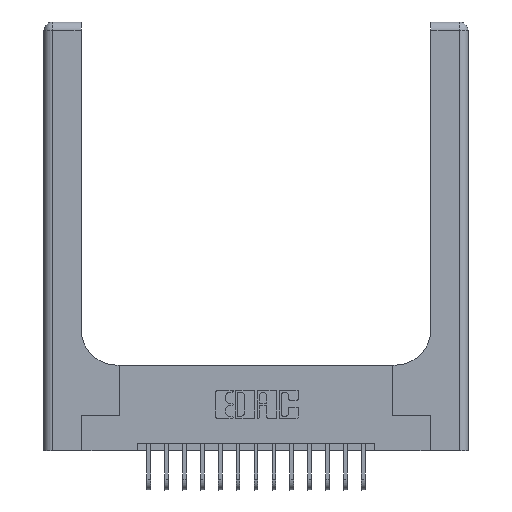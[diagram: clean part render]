
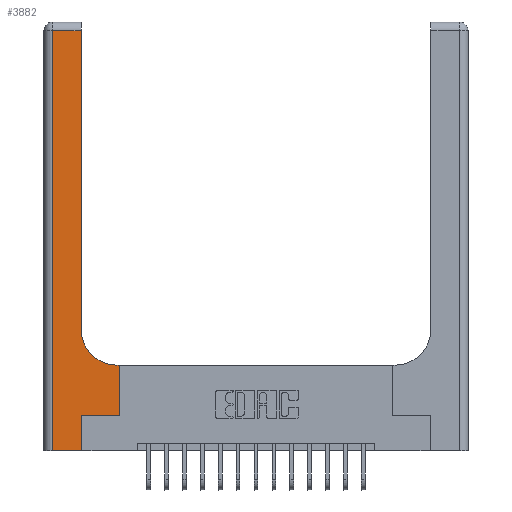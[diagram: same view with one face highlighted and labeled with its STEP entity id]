
A CAD part, top view. The second image highlights one B-rep face of the part: STEP entity #3882.
In plain terms, the highlighted planar face has unit normal (0, 0, 1).
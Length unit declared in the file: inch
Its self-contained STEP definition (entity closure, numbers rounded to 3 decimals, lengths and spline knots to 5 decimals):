
#347 = LINE ( 'NONE', #11048, #7003 ) ;
#745 = DIRECTION ( 'NONE',  ( 0., 0., -1. ) ) ;
#1070 = VERTEX_POINT ( 'NONE', #12619 ) ;
#1079 = VERTEX_POINT ( 'NONE', #16019 ) ;
#1255 = DIRECTION ( 'NONE',  ( 0., 1., 0. ) ) ;
#1820 = DIRECTION ( 'NONE',  ( 0., 0., -1. ) ) ;
#1949 = VECTOR ( 'NONE', #17035, 39.37008 ) ;
#2399 = CARTESIAN_POINT ( 'NONE',  ( 0.265, 0., 0.37 ) ) ;
#2413 = CARTESIAN_POINT ( 'NONE',  ( 0.06, 0., 0.37 ) ) ;
#2443 = EDGE_CURVE ( 'NONE', #8974, #7378, #15107, .T. ) ;
#2961 = DIRECTION ( 'NONE',  ( 0., 1., 0. ) ) ;
#3458 = DIRECTION ( 'NONE',  ( 0., -1., 0. ) ) ;
#3665 = EDGE_CURVE ( 'NONE', #13594, #1070, #16737, .T. ) ;
#3882 = ADVANCED_FACE ( 'NONE', ( #6750 ), #15320, .F. ) ;
#3956 = VECTOR ( 'NONE', #4130, 39.37008 ) ;
#4108 = ORIENTED_EDGE ( 'NONE', *, *, #6225, .T. ) ;
#4130 = DIRECTION ( 'NONE',  ( 1., 0., 0. ) ) ;
#4310 = EDGE_CURVE ( 'NONE', #1079, #11461, #16512, .T. ) ;
#4519 = ORIENTED_EDGE ( 'NONE', *, *, #4310, .T. ) ;
#4709 = ORIENTED_EDGE ( 'NONE', *, *, #11155, .T. ) ;
#5202 = EDGE_CURVE ( 'NONE', #15884, #7042, #11118, .T. ) ;
#5296 = AXIS2_PLACEMENT_3D ( 'NONE', #7367, #745, #10072 ) ;
#5558 = ORIENTED_EDGE ( 'NONE', *, *, #5202, .T. ) ;
#6225 = EDGE_CURVE ( 'NONE', #1070, #1079, #11086, .T. ) ;
#6324 = CARTESIAN_POINT ( 'NONE',  ( 0.26, 0.85, 0.37 ) ) ;
#6667 = VECTOR ( 'NONE', #8666, 39.37008 ) ;
#6750 = FACE_OUTER_BOUND ( 'NONE', #10823, .T. ) ;
#6798 = ORIENTED_EDGE ( 'NONE', *, *, #9149, .T. ) ;
#7003 = VECTOR ( 'NONE', #12362, 39.37008 ) ;
#7042 = VERTEX_POINT ( 'NONE', #2413 ) ;
#7367 = CARTESIAN_POINT ( 'NONE',  ( 0., 3., 0.37 ) ) ;
#7378 = VERTEX_POINT ( 'NONE', #12519 ) ;
#7526 = VECTOR ( 'NONE', #3458, 39.37008 ) ;
#8053 = VECTOR ( 'NONE', #1255, 39.37008 ) ;
#8268 = CARTESIAN_POINT ( 'NONE',  ( 0.528, 0.25, 0.37 ) ) ;
#8422 = CARTESIAN_POINT ( 'NONE',  ( 0.06, 2.94, 0.37 ) ) ;
#8666 = DIRECTION ( 'NONE',  ( -1., 0., 0. ) ) ;
#8974 = VERTEX_POINT ( 'NONE', #2399 ) ;
#9086 = CARTESIAN_POINT ( 'NONE',  ( 0., 0., 0.37 ) ) ;
#9149 = EDGE_CURVE ( 'NONE', #7378, #13594, #14131, .T. ) ;
#9816 = CARTESIAN_POINT ( 'NONE',  ( 0.51, 0.85, 0.37 ) ) ;
#10072 = DIRECTION ( 'NONE',  ( -1., 0., 0. ) ) ;
#10255 = VERTEX_POINT ( 'NONE', #16000 ) ;
#10607 = EDGE_CURVE ( 'NONE', #10255, #15884, #347, .T. ) ;
#10615 = CARTESIAN_POINT ( 'NONE',  ( 0.265, 0., 0.37 ) ) ;
#10823 = EDGE_LOOP ( 'NONE', ( #4709, #15743, #5558, #13059, #16574, #6798, #14280, #4108, #4519 ) ) ;
#11048 = CARTESIAN_POINT ( 'NONE',  ( 0., 2.94, 0.37 ) ) ;
#11086 = LINE ( 'NONE', #13944, #6667 ) ;
#11118 = LINE ( 'NONE', #16694, #7526 ) ;
#11155 = EDGE_CURVE ( 'NONE', #11461, #10255, #12835, .T. ) ;
#11175 = DIRECTION ( 'NONE',  ( 1., 0., 0. ) ) ;
#11461 = VERTEX_POINT ( 'NONE', #6324 ) ;
#12117 = CARTESIAN_POINT ( 'NONE',  ( 0.265, 0.25, 0.37 ) ) ;
#12124 = AXIS2_PLACEMENT_3D ( 'NONE', #9816, #1820, #11175 ) ;
#12362 = DIRECTION ( 'NONE',  ( -1., 0., 0. ) ) ;
#12519 = CARTESIAN_POINT ( 'NONE',  ( 0.265, 0.25, 0.37 ) ) ;
#12619 = CARTESIAN_POINT ( 'NONE',  ( 0.528, 0.6, 0.37 ) ) ;
#12835 = LINE ( 'NONE', #13605, #15508 ) ;
#13059 = ORIENTED_EDGE ( 'NONE', *, *, #13138, .T. ) ;
#13138 = EDGE_CURVE ( 'NONE', #7042, #8974, #16109, .T. ) ;
#13220 = VECTOR ( 'NONE', #2961, 39.37008 ) ;
#13594 = VERTEX_POINT ( 'NONE', #13992 ) ;
#13605 = CARTESIAN_POINT ( 'NONE',  ( 0.26, 3., 0.37 ) ) ;
#13944 = CARTESIAN_POINT ( 'NONE',  ( 0.26, 0.6, 0.37 ) ) ;
#13992 = CARTESIAN_POINT ( 'NONE',  ( 0.528, 0.25, 0.37 ) ) ;
#14131 = LINE ( 'NONE', #12117, #3956 ) ;
#14280 = ORIENTED_EDGE ( 'NONE', *, *, #3665, .T. ) ;
#14918 = DIRECTION ( 'NONE',  ( 0., 1., 0. ) ) ;
#15107 = LINE ( 'NONE', #10615, #8053 ) ;
#15320 = PLANE ( 'NONE',  #5296 ) ;
#15508 = VECTOR ( 'NONE', #14918, 39.37008 ) ;
#15743 = ORIENTED_EDGE ( 'NONE', *, *, #10607, .T. ) ;
#15884 = VERTEX_POINT ( 'NONE', #8422 ) ;
#16000 = CARTESIAN_POINT ( 'NONE',  ( 0.26, 2.94, 0.37 ) ) ;
#16019 = CARTESIAN_POINT ( 'NONE',  ( 0.51, 0.6, 0.37 ) ) ;
#16109 = LINE ( 'NONE', #9086, #1949 ) ;
#16512 = CIRCLE ( 'NONE', #12124, 0.25 ) ;
#16574 = ORIENTED_EDGE ( 'NONE', *, *, #2443, .T. ) ;
#16694 = CARTESIAN_POINT ( 'NONE',  ( 0.06, 3., 0.37 ) ) ;
#16737 = LINE ( 'NONE', #8268, #13220 ) ;
#17035 = DIRECTION ( 'NONE',  ( 1., 0., 0. ) ) ;
